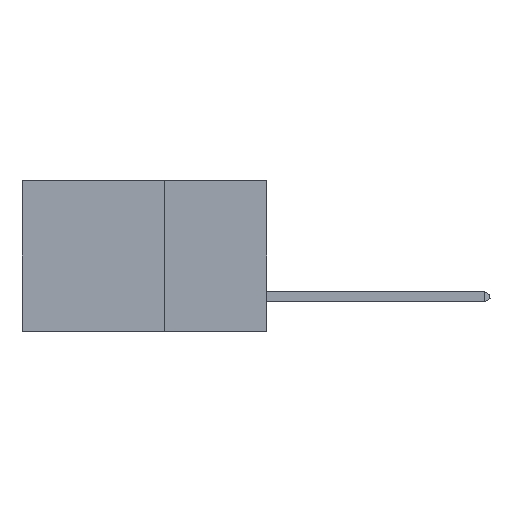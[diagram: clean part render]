
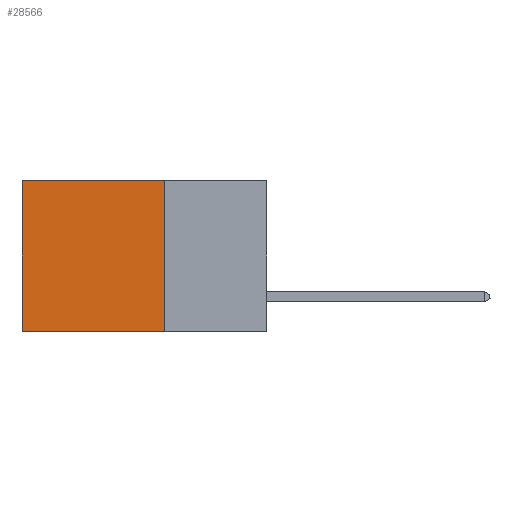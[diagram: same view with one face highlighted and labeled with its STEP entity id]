
A CAD part, left-side view. The second image highlights one B-rep face of the part: STEP entity #28566.
In plain terms, the highlighted planar face has unit normal (-1, 0, 0).
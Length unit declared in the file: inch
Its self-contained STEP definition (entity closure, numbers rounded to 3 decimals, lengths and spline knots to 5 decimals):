
#1846 = LINE ( 'NONE', #2584, #10635 ) ;
#1935 = AXIS2_PLACEMENT_3D ( 'NONE', #28481, #35113, #8866 ) ;
#1966 = CARTESIAN_POINT ( 'NONE',  ( 0.2875, 0.25, 0. ) ) ;
#2584 = CARTESIAN_POINT ( 'NONE',  ( 0.2875, 0.6, 0. ) ) ;
#3201 = ORIENTED_EDGE ( 'NONE', *, *, #36543, .F. ) ;
#4810 = VECTOR ( 'NONE', #11516, 39.37008 ) ;
#6776 = ORIENTED_EDGE ( 'NONE', *, *, #21829, .T. ) ;
#6863 = LINE ( 'NONE', #1966, #4810 ) ;
#8866 = DIRECTION ( 'NONE',  ( 0., 0., -1. ) ) ;
#10169 = EDGE_CURVE ( 'NONE', #28377, #12276, #25299, .T. ) ;
#10635 = VECTOR ( 'NONE', #42261, 39.37008 ) ;
#11516 = DIRECTION ( 'NONE',  ( 0., 1., 0. ) ) ;
#12276 = VERTEX_POINT ( 'NONE', #25995 ) ;
#13385 = VERTEX_POINT ( 'NONE', #22500 ) ;
#18100 = DIRECTION ( 'NONE',  ( 0., 1., 0. ) ) ;
#18555 = PLANE ( 'NONE',  #1935 ) ;
#21258 = FACE_OUTER_BOUND ( 'NONE', #29809, .T. ) ;
#21829 = EDGE_CURVE ( 'NONE', #13385, #12276, #1846, .T. ) ;
#22500 = CARTESIAN_POINT ( 'NONE',  ( 0.2875, 0.6, 0. ) ) ;
#25299 = LINE ( 'NONE', #26571, #26338 ) ;
#25995 = CARTESIAN_POINT ( 'NONE',  ( 0.2875, 0.6, -0.37 ) ) ;
#26338 = VECTOR ( 'NONE', #18100, 39.37008 ) ;
#26571 = CARTESIAN_POINT ( 'NONE',  ( 0.2875, 0.25, -0.37 ) ) ;
#27984 = EDGE_CURVE ( 'NONE', #37660, #13385, #6863, .T. ) ;
#28377 = VERTEX_POINT ( 'NONE', #30688 ) ;
#28481 = CARTESIAN_POINT ( 'NONE',  ( 0.2875, 0.25, 0. ) ) ;
#28566 = ADVANCED_FACE ( 'NONE', ( #21258 ), #18555, .F. ) ;
#29809 = EDGE_LOOP ( 'NONE', ( #6776, #41795, #3201, #30588 ) ) ;
#30588 = ORIENTED_EDGE ( 'NONE', *, *, #27984, .T. ) ;
#30688 = CARTESIAN_POINT ( 'NONE',  ( 0.2875, 0.25, -0.37 ) ) ;
#30722 = CARTESIAN_POINT ( 'NONE',  ( 0.2875, 0.25, 0. ) ) ;
#33439 = CARTESIAN_POINT ( 'NONE',  ( 0.2875, 0.25, 0. ) ) ;
#33497 = VECTOR ( 'NONE', #40073, 39.37008 ) ;
#35113 = DIRECTION ( 'NONE',  ( 1., 0., 0. ) ) ;
#36543 = EDGE_CURVE ( 'NONE', #37660, #28377, #39147, .T. ) ;
#37660 = VERTEX_POINT ( 'NONE', #30722 ) ;
#39147 = LINE ( 'NONE', #33439, #33497 ) ;
#40073 = DIRECTION ( 'NONE',  ( 0., 0., -1. ) ) ;
#41795 = ORIENTED_EDGE ( 'NONE', *, *, #10169, .F. ) ;
#42261 = DIRECTION ( 'NONE',  ( 0., 0., -1. ) ) ;
